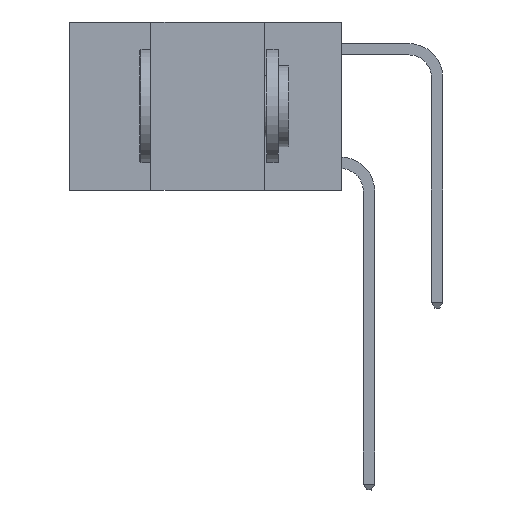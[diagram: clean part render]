
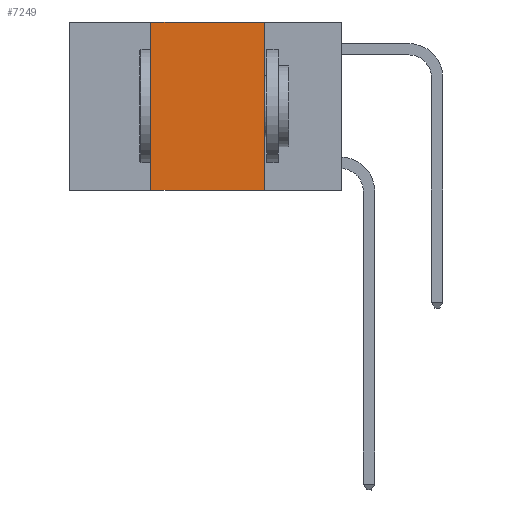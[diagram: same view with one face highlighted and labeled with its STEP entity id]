
A CAD part, left-side view. The second image highlights one B-rep face of the part: STEP entity #7249.
In plain terms, the highlighted planar face has unit normal (-1, 0, 0).
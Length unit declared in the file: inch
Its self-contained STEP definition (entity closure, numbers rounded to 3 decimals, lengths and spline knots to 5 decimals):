
#903 = DIRECTION ( 'NONE',  ( 1., 0., 0. ) ) ;
#1424 = VECTOR ( 'NONE', #3279, 39.37008 ) ;
#1745 = CARTESIAN_POINT ( 'NONE',  ( 0., 0.42, -0.37 ) ) ;
#1785 = ORIENTED_EDGE ( 'NONE', *, *, #3972, .F. ) ;
#2054 = CARTESIAN_POINT ( 'NONE',  ( 0., 0.42, 0. ) ) ;
#2151 = VERTEX_POINT ( 'NONE', #12278 ) ;
#2173 = DIRECTION ( 'NONE',  ( 0., -1., 0. ) ) ;
#2221 = FACE_OUTER_BOUND ( 'NONE', #6116, .T. ) ;
#2541 = DIRECTION ( 'NONE',  ( 0., -1., 0. ) ) ;
#2570 = VERTEX_POINT ( 'NONE', #1745 ) ;
#3279 = DIRECTION ( 'NONE',  ( 0., 0., 1. ) ) ;
#3331 = CARTESIAN_POINT ( 'NONE',  ( 0., 0.6, -0.37 ) ) ;
#3735 = VECTOR ( 'NONE', #6553, 39.37008 ) ;
#3972 = EDGE_CURVE ( 'NONE', #9978, #2151, #4115, .T. ) ;
#4115 = LINE ( 'NONE', #12101, #3735 ) ;
#5231 = VECTOR ( 'NONE', #2173, 39.37008 ) ;
#5612 = LINE ( 'NONE', #3331, #5231 ) ;
#6116 = EDGE_LOOP ( 'NONE', ( #1785, #6296, #12349, #12594 ) ) ;
#6264 = CARTESIAN_POINT ( 'NONE',  ( 0., 0.42, 0. ) ) ;
#6296 = ORIENTED_EDGE ( 'NONE', *, *, #10640, .F. ) ;
#6377 = VECTOR ( 'NONE', #2541, 39.37008 ) ;
#6553 = DIRECTION ( 'NONE',  ( 0., 0., -1. ) ) ;
#7249 = ADVANCED_FACE ( 'NONE', ( #2221 ), #14749, .F. ) ;
#7773 = EDGE_CURVE ( 'NONE', #2570, #8799, #9654, .T. ) ;
#8799 = VERTEX_POINT ( 'NONE', #6264 ) ;
#9133 = DIRECTION ( 'NONE',  ( 0., 0., -1. ) ) ;
#9446 = CARTESIAN_POINT ( 'NONE',  ( 0., 0.17, 0. ) ) ;
#9513 = CARTESIAN_POINT ( 'NONE',  ( 0., 0.6, 0. ) ) ;
#9654 = LINE ( 'NONE', #2054, #1424 ) ;
#9774 = AXIS2_PLACEMENT_3D ( 'NONE', #10183, #903, #9133 ) ;
#9978 = VERTEX_POINT ( 'NONE', #9446 ) ;
#10183 = CARTESIAN_POINT ( 'NONE',  ( 0., 0.6, 0. ) ) ;
#10640 = EDGE_CURVE ( 'NONE', #8799, #9978, #14987, .T. ) ;
#11096 = EDGE_CURVE ( 'NONE', #2570, #2151, #5612, .T. ) ;
#12101 = CARTESIAN_POINT ( 'NONE',  ( 0., 0.17, 0. ) ) ;
#12278 = CARTESIAN_POINT ( 'NONE',  ( 0., 0.17, -0.37 ) ) ;
#12349 = ORIENTED_EDGE ( 'NONE', *, *, #7773, .F. ) ;
#12594 = ORIENTED_EDGE ( 'NONE', *, *, #11096, .T. ) ;
#14749 = PLANE ( 'NONE',  #9774 ) ;
#14987 = LINE ( 'NONE', #9513, #6377 ) ;
